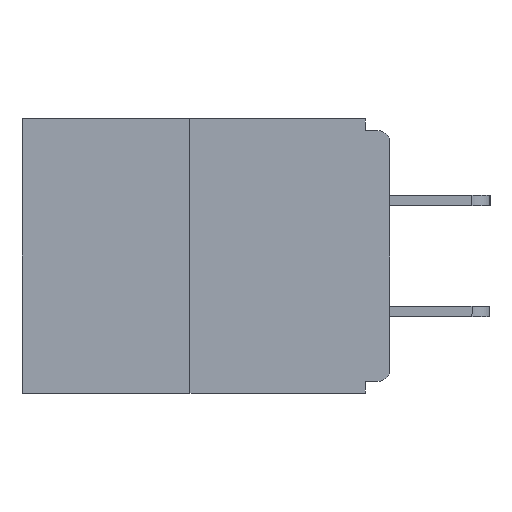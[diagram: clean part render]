
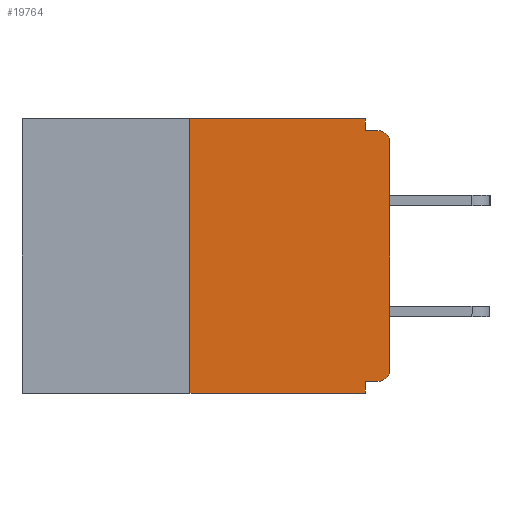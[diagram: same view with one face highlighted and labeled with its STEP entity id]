
A CAD part, left-side view. The second image highlights one B-rep face of the part: STEP entity #19764.
In plain terms, the highlighted planar face has unit normal (-1, 0, 0).
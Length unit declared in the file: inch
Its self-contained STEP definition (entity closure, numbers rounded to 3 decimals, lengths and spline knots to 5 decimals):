
#148 = DIRECTION ( 'NONE',  ( 0., -1., 0. ) ) ;
#170 = ORIENTED_EDGE ( 'NONE', *, *, #16725, .T. ) ;
#305 = CARTESIAN_POINT ( 'NONE',  ( 0., 0.031, 0. ) ) ;
#358 = DIRECTION ( 'NONE',  ( 0., 0., -1. ) ) ;
#571 = VECTOR ( 'NONE', #14613, 39.37008 ) ;
#577 = EDGE_CURVE ( 'NONE', #20422, #17907, #4822, .T. ) ;
#698 = EDGE_CURVE ( 'NONE', #21314, #20422, #15063, .T. ) ;
#797 = CARTESIAN_POINT ( 'NONE',  ( 0., 0.25, 0. ) ) ;
#894 = ORIENTED_EDGE ( 'NONE', *, *, #577, .T. ) ;
#972 = VECTOR ( 'NONE', #15160, 39.37008 ) ;
#1454 = ORIENTED_EDGE ( 'NONE', *, *, #7074, .F. ) ;
#2481 = CARTESIAN_POINT ( 'NONE',  ( 0., 0.25, -0.343 ) ) ;
#2756 = VERTEX_POINT ( 'NONE', #2481 ) ;
#3102 = ORIENTED_EDGE ( 'NONE', *, *, #698, .T. ) ;
#3239 = VERTEX_POINT ( 'NONE', #7750 ) ;
#3520 = VECTOR ( 'NONE', #8269, 39.37008 ) ;
#3836 = CARTESIAN_POINT ( 'NONE',  ( 0., 0.031, -0.343 ) ) ;
#3992 = DIRECTION ( 'NONE',  ( 0., 1., 0. ) ) ;
#4714 = VECTOR ( 'NONE', #7562, 39.37008 ) ;
#4822 = CIRCLE ( 'NONE', #25182, 0.015 ) ;
#5350 = CARTESIAN_POINT ( 'NONE',  ( 0., 0.46, 0. ) ) ;
#5535 = CARTESIAN_POINT ( 'NONE',  ( 0., 0.25, 0. ) ) ;
#6453 = EDGE_CURVE ( 'NONE', #2756, #24282, #25252, .T. ) ;
#7074 = EDGE_CURVE ( 'NONE', #20440, #9245, #24240, .T. ) ;
#7105 = DIRECTION ( 'NONE',  ( 0., 0., 1. ) ) ;
#7165 = VERTEX_POINT ( 'NONE', #15019 ) ;
#7363 = LINE ( 'NONE', #21156, #972 ) ;
#7562 = DIRECTION ( 'NONE',  ( 0., -1., 0. ) ) ;
#7649 = PLANE ( 'NONE',  #11706 ) ;
#7750 = CARTESIAN_POINT ( 'NONE',  ( 0., 0.031, 0. ) ) ;
#8269 = DIRECTION ( 'NONE',  ( 0., 0., 1. ) ) ;
#8575 = DIRECTION ( 'NONE',  ( -1., 0., 0. ) ) ;
#9079 = ORIENTED_EDGE ( 'NONE', *, *, #6453, .F. ) ;
#9245 = VERTEX_POINT ( 'NONE', #25517 ) ;
#10166 = VECTOR ( 'NONE', #7105, 39.37008 ) ;
#10489 = LINE ( 'NONE', #305, #571 ) ;
#10938 = VECTOR ( 'NONE', #3992, 39.37008 ) ;
#11240 = LINE ( 'NONE', #20277, #10938 ) ;
#11706 = AXIS2_PLACEMENT_3D ( 'NONE', #5350, #21728, #22456 ) ;
#11924 = DIRECTION ( 'NONE',  ( -1., 0., 0. ) ) ;
#12362 = CARTESIAN_POINT ( 'NONE',  ( 0., 0., 0. ) ) ;
#12448 = EDGE_CURVE ( 'NONE', #19213, #17907, #7363, .T. ) ;
#12589 = ORIENTED_EDGE ( 'NONE', *, *, #24975, .F. ) ;
#13075 = CARTESIAN_POINT ( 'NONE',  ( 0., 0., -0.313 ) ) ;
#14001 = ORIENTED_EDGE ( 'NONE', *, *, #12448, .F. ) ;
#14091 = DIRECTION ( 'NONE',  ( 0., 0., -1. ) ) ;
#14144 = EDGE_LOOP ( 'NONE', ( #15998, #9079, #170, #1454, #12589, #26531, #3102, #894, #14001, #24422 ) ) ;
#14364 = VECTOR ( 'NONE', #148, 39.37008 ) ;
#14474 = CARTESIAN_POINT ( 'NONE',  ( 0., 0.015, -0.313 ) ) ;
#14613 = DIRECTION ( 'NONE',  ( 0., 0., -1. ) ) ;
#15019 = CARTESIAN_POINT ( 'NONE',  ( 0., 0.015, -0.328 ) ) ;
#15063 = LINE ( 'NONE', #12362, #3520 ) ;
#15160 = DIRECTION ( 'NONE',  ( 0., -1., 0. ) ) ;
#15639 = LINE ( 'NONE', #24696, #14364 ) ;
#15957 = CARTESIAN_POINT ( 'NONE',  ( 0., 0., -0.03 ) ) ;
#15998 = ORIENTED_EDGE ( 'NONE', *, *, #20869, .F. ) ;
#16152 = CARTESIAN_POINT ( 'NONE',  ( 0., 0.031, -0.015 ) ) ;
#16318 = CARTESIAN_POINT ( 'NONE',  ( 0., 0.031, -0.328 ) ) ;
#16725 = EDGE_CURVE ( 'NONE', #2756, #9245, #15639, .T. ) ;
#17584 = CIRCLE ( 'NONE', #20241, 0.015 ) ;
#17907 = VERTEX_POINT ( 'NONE', #18273 ) ;
#18273 = CARTESIAN_POINT ( 'NONE',  ( 0., 0.015, -0.015 ) ) ;
#18777 = VECTOR ( 'NONE', #22114, 39.37008 ) ;
#19121 = LINE ( 'NONE', #23724, #4714 ) ;
#19213 = VERTEX_POINT ( 'NONE', #16152 ) ;
#19764 = ADVANCED_FACE ( 'NONE', ( #24014 ), #7649, .F. ) ;
#20241 = AXIS2_PLACEMENT_3D ( 'NONE', #14474, #8575, #358 ) ;
#20277 = CARTESIAN_POINT ( 'NONE',  ( 0., 0., -0.328 ) ) ;
#20422 = VERTEX_POINT ( 'NONE', #15957 ) ;
#20440 = VERTEX_POINT ( 'NONE', #16318 ) ;
#20699 = EDGE_CURVE ( 'NONE', #3239, #19213, #10489, .T. ) ;
#20869 = EDGE_CURVE ( 'NONE', #24282, #3239, #19121, .T. ) ;
#21156 = CARTESIAN_POINT ( 'NONE',  ( 0., 0., -0.015 ) ) ;
#21314 = VERTEX_POINT ( 'NONE', #13075 ) ;
#21728 = DIRECTION ( 'NONE',  ( 1., 0., 0. ) ) ;
#22114 = DIRECTION ( 'NONE',  ( 0., 0., -1. ) ) ;
#22348 = CARTESIAN_POINT ( 'NONE',  ( 0., 0.015, -0.03 ) ) ;
#22456 = DIRECTION ( 'NONE',  ( 0., 0., -1. ) ) ;
#23724 = CARTESIAN_POINT ( 'NONE',  ( 0., 0.46, 0. ) ) ;
#24014 = FACE_OUTER_BOUND ( 'NONE', #14144, .T. ) ;
#24240 = LINE ( 'NONE', #3836, #18777 ) ;
#24282 = VERTEX_POINT ( 'NONE', #5535 ) ;
#24422 = ORIENTED_EDGE ( 'NONE', *, *, #20699, .F. ) ;
#24696 = CARTESIAN_POINT ( 'NONE',  ( 0., 0.46, -0.343 ) ) ;
#24975 = EDGE_CURVE ( 'NONE', #7165, #20440, #11240, .T. ) ;
#25182 = AXIS2_PLACEMENT_3D ( 'NONE', #22348, #11924, #14091 ) ;
#25252 = LINE ( 'NONE', #797, #10166 ) ;
#25517 = CARTESIAN_POINT ( 'NONE',  ( 0., 0.031, -0.343 ) ) ;
#26432 = EDGE_CURVE ( 'NONE', #7165, #21314, #17584, .T. ) ;
#26531 = ORIENTED_EDGE ( 'NONE', *, *, #26432, .T. ) ;
